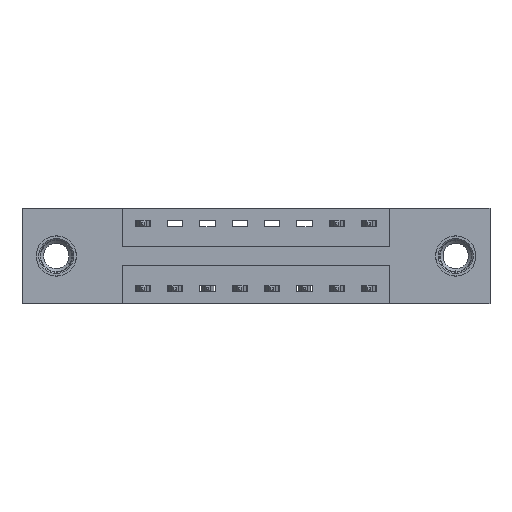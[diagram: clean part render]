
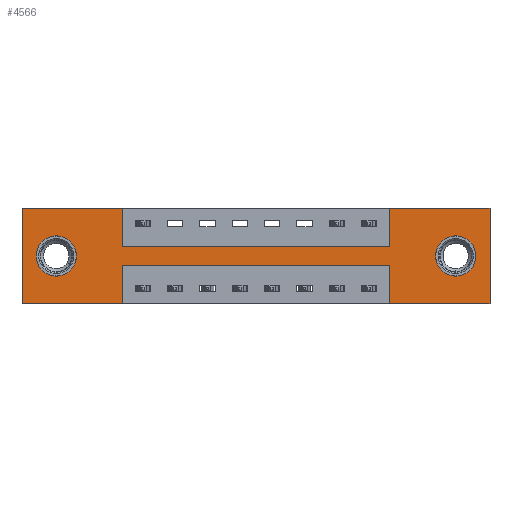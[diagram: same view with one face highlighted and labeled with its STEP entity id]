
A CAD part, front view. The second image highlights one B-rep face of the part: STEP entity #4566.
In plain terms, the highlighted planar face has unit normal (0, -1, 0).
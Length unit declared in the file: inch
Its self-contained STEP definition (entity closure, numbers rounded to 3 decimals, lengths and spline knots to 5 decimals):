
#24 = DIRECTION ( 'NONE',  ( 0., 0., -1. ) ) ;
#69 = DIRECTION ( 'NONE',  ( 0., 0., 1. ) ) ;
#92 = EDGE_CURVE ( 'NONE', #4048, #4417, #8899, .T. ) ;
#182 = CARTESIAN_POINT ( 'NONE',  ( 1.4225, 0., -0.15 ) ) ;
#255 = ORIENTED_EDGE ( 'NONE', *, *, #9028, .F. ) ;
#522 = VECTOR ( 'NONE', #6931, 39.37008 ) ;
#584 = VERTEX_POINT ( 'NONE', #8476 ) ;
#588 = DIRECTION ( 'NONE',  ( 0., 0., -1. ) ) ;
#597 = CARTESIAN_POINT ( 'NONE',  ( 1.6775, 0., -0.107 ) ) ;
#667 = ORIENTED_EDGE ( 'NONE', *, *, #2666, .F. ) ;
#691 = DIRECTION ( 'NONE',  ( 0., 0., 1. ) ) ;
#806 = DIRECTION ( 'NONE',  ( -1., 0., 0. ) ) ;
#878 = CARTESIAN_POINT ( 'NONE',  ( 0.1325, 0., -0.185 ) ) ;
#986 = FACE_OUTER_BOUND ( 'NONE', #8936, .T. ) ;
#999 = CARTESIAN_POINT ( 'NONE',  ( 1.4225, 0., -0.37 ) ) ;
#1041 = DIRECTION ( 'NONE',  ( -1., 0., 0. ) ) ;
#1147 = VERTEX_POINT ( 'NONE', #4420 ) ;
#1195 = DIRECTION ( 'NONE',  ( 1., 0., 0. ) ) ;
#1270 = CARTESIAN_POINT ( 'NONE',  ( 1.4225, 0., 0. ) ) ;
#1328 = LINE ( 'NONE', #5166, #9951 ) ;
#1451 = LINE ( 'NONE', #9693, #5874 ) ;
#1571 = FACE_BOUND ( 'NONE', #4125, .T. ) ;
#1792 = DIRECTION ( 'NONE',  ( 0., 0., 1. ) ) ;
#1912 = CARTESIAN_POINT ( 'NONE',  ( 1.81, 0., 0. ) ) ;
#1940 = VERTEX_POINT ( 'NONE', #2311 ) ;
#1969 = DIRECTION ( 'NONE',  ( 0., -1., 0. ) ) ;
#1970 = ORIENTED_EDGE ( 'NONE', *, *, #4651, .F. ) ;
#2231 = DIRECTION ( 'NONE',  ( 0., 0., -1. ) ) ;
#2251 = ORIENTED_EDGE ( 'NONE', *, *, #8188, .F. ) ;
#2311 = CARTESIAN_POINT ( 'NONE',  ( 0.1325, 0., -0.107 ) ) ;
#2666 = EDGE_CURVE ( 'NONE', #3934, #1147, #8643, .T. ) ;
#2674 = CARTESIAN_POINT ( 'NONE',  ( 0., 0., 0. ) ) ;
#2688 = CARTESIAN_POINT ( 'NONE',  ( 1.81, 0., 0. ) ) ;
#3094 = ORIENTED_EDGE ( 'NONE', *, *, #8072, .T. ) ;
#3206 = EDGE_CURVE ( 'NONE', #584, #7445, #9226, .T. ) ;
#3356 = AXIS2_PLACEMENT_3D ( 'NONE', #878, #6961, #1792 ) ;
#3616 = DIRECTION ( 'NONE',  ( 0., 0., -1. ) ) ;
#3652 = EDGE_CURVE ( 'NONE', #1147, #9329, #4982, .T. ) ;
#3721 = VERTEX_POINT ( 'NONE', #182 ) ;
#3740 = ORIENTED_EDGE ( 'NONE', *, *, #92, .F. ) ;
#3747 = AXIS2_PLACEMENT_3D ( 'NONE', #10166, #5443, #69 ) ;
#3749 = LINE ( 'NONE', #9170, #8137 ) ;
#3753 = CARTESIAN_POINT ( 'NONE',  ( 0.3875, 0., -0.22 ) ) ;
#3787 = CARTESIAN_POINT ( 'NONE',  ( 0., 0., -0.37 ) ) ;
#3835 = VERTEX_POINT ( 'NONE', #5760 ) ;
#3934 = VERTEX_POINT ( 'NONE', #8374 ) ;
#4048 = VERTEX_POINT ( 'NONE', #1912 ) ;
#4081 = VECTOR ( 'NONE', #3616, 39.37008 ) ;
#4125 = EDGE_LOOP ( 'NONE', ( #9941, #8256 ) ) ;
#4154 = CIRCLE ( 'NONE', #3747, 0.078 ) ;
#4271 = DIRECTION ( 'NONE',  ( 0., 1., 0. ) ) ;
#4306 = VECTOR ( 'NONE', #7866, 39.37008 ) ;
#4415 = CARTESIAN_POINT ( 'NONE',  ( 1.81, 0., -0.37 ) ) ;
#4417 = VERTEX_POINT ( 'NONE', #4415 ) ;
#4420 = CARTESIAN_POINT ( 'NONE',  ( 0.3875, 0., 0. ) ) ;
#4431 = VECTOR ( 'NONE', #24, 39.37008 ) ;
#4566 = ADVANCED_FACE ( 'NONE', ( #5719, #1571, #986 ), #9475, .T. ) ;
#4651 = EDGE_CURVE ( 'NONE', #3721, #7153, #6582, .T. ) ;
#4714 = DIRECTION ( 'NONE',  ( 1., 0., 0. ) ) ;
#4905 = ORIENTED_EDGE ( 'NONE', *, *, #5644, .F. ) ;
#4982 = LINE ( 'NONE', #9378, #4431 ) ;
#5100 = EDGE_LOOP ( 'NONE', ( #6902, #3094 ) ) ;
#5166 = CARTESIAN_POINT ( 'NONE',  ( 0., 0., -0.37 ) ) ;
#5443 = DIRECTION ( 'NONE',  ( 0., 1., 0. ) ) ;
#5510 = VECTOR ( 'NONE', #806, 39.37008 ) ;
#5639 = CARTESIAN_POINT ( 'NONE',  ( 0.3875, 0., -0.15 ) ) ;
#5644 = EDGE_CURVE ( 'NONE', #7153, #4048, #7439, .T. ) ;
#5719 = FACE_BOUND ( 'NONE', #5100, .T. ) ;
#5760 = CARTESIAN_POINT ( 'NONE',  ( 0.3875, 0., -0.37 ) ) ;
#5811 = ORIENTED_EDGE ( 'NONE', *, *, #10298, .F. ) ;
#5830 = ORIENTED_EDGE ( 'NONE', *, *, #3652, .F. ) ;
#5874 = VECTOR ( 'NONE', #2231, 39.37008 ) ;
#5878 = AXIS2_PLACEMENT_3D ( 'NONE', #3787, #1969, #7925 ) ;
#5919 = DIRECTION ( 'NONE',  ( 0., 1., 0. ) ) ;
#5929 = CARTESIAN_POINT ( 'NONE',  ( 1.4225, 0., 0. ) ) ;
#5945 = EDGE_CURVE ( 'NONE', #9329, #3721, #7047, .T. ) ;
#6000 = ORIENTED_EDGE ( 'NONE', *, *, #5945, .F. ) ;
#6213 = EDGE_CURVE ( 'NONE', #9638, #8257, #8794, .T. ) ;
#6582 = LINE ( 'NONE', #1270, #6834 ) ;
#6834 = VECTOR ( 'NONE', #7292, 39.37008 ) ;
#6902 = ORIENTED_EDGE ( 'NONE', *, *, #6213, .T. ) ;
#6931 = DIRECTION ( 'NONE',  ( 1., 0., 0. ) ) ;
#6961 = DIRECTION ( 'NONE',  ( 0., 1., 0. ) ) ;
#7005 = CIRCLE ( 'NONE', #7142, 0.078 ) ;
#7047 = LINE ( 'NONE', #5639, #8924 ) ;
#7110 = VECTOR ( 'NONE', #1041, 39.37008 ) ;
#7142 = AXIS2_PLACEMENT_3D ( 'NONE', #9103, #4271, #9871 ) ;
#7153 = VERTEX_POINT ( 'NONE', #5929 ) ;
#7172 = CARTESIAN_POINT ( 'NONE',  ( 0.3875, 0., -0.15 ) ) ;
#7292 = DIRECTION ( 'NONE',  ( 0., 0., 1. ) ) ;
#7439 = LINE ( 'NONE', #2674, #522 ) ;
#7445 = VERTEX_POINT ( 'NONE', #7760 ) ;
#7760 = CARTESIAN_POINT ( 'NONE',  ( 0.3875, 0., -0.22 ) ) ;
#7765 = CARTESIAN_POINT ( 'NONE',  ( 1.4225, 0., -0.37 ) ) ;
#7866 = DIRECTION ( 'NONE',  ( 0., 0., 1. ) ) ;
#7925 = DIRECTION ( 'NONE',  ( 0., 0., -1. ) ) ;
#8072 = EDGE_CURVE ( 'NONE', #8257, #9638, #7005, .T. ) ;
#8137 = VECTOR ( 'NONE', #691, 39.37008 ) ;
#8165 = EDGE_CURVE ( 'NONE', #3835, #9545, #1328, .T. ) ;
#8188 = EDGE_CURVE ( 'NONE', #9545, #3934, #3749, .T. ) ;
#8256 = ORIENTED_EDGE ( 'NONE', *, *, #10789, .T. ) ;
#8257 = VERTEX_POINT ( 'NONE', #9228 ) ;
#8342 = ORIENTED_EDGE ( 'NONE', *, *, #8165, .F. ) ;
#8374 = CARTESIAN_POINT ( 'NONE',  ( 0., 0., 0. ) ) ;
#8476 = CARTESIAN_POINT ( 'NONE',  ( 1.4225, 0., -0.22 ) ) ;
#8643 = LINE ( 'NONE', #10262, #8877 ) ;
#8794 = CIRCLE ( 'NONE', #10361, 0.078 ) ;
#8859 = LINE ( 'NONE', #999, #4306 ) ;
#8877 = VECTOR ( 'NONE', #4714, 39.37008 ) ;
#8899 = LINE ( 'NONE', #2688, #4081 ) ;
#8924 = VECTOR ( 'NONE', #1195, 39.37008 ) ;
#8936 = EDGE_LOOP ( 'NONE', ( #5811, #9159, #9221, #255, #3740, #4905, #1970, #6000, #5830, #667, #2251, #8342 ) ) ;
#8990 = VERTEX_POINT ( 'NONE', #10634 ) ;
#9028 = EDGE_CURVE ( 'NONE', #4417, #9861, #9708, .T. ) ;
#9103 = CARTESIAN_POINT ( 'NONE',  ( 1.6775, 0., -0.185 ) ) ;
#9159 = ORIENTED_EDGE ( 'NONE', *, *, #3206, .F. ) ;
#9170 = CARTESIAN_POINT ( 'NONE',  ( 0., 0., 0. ) ) ;
#9221 = ORIENTED_EDGE ( 'NONE', *, *, #9969, .F. ) ;
#9226 = LINE ( 'NONE', #3753, #7110 ) ;
#9228 = CARTESIAN_POINT ( 'NONE',  ( 1.6775, 0., -0.263 ) ) ;
#9329 = VERTEX_POINT ( 'NONE', #7172 ) ;
#9378 = CARTESIAN_POINT ( 'NONE',  ( 0.3875, 0., 0. ) ) ;
#9475 = PLANE ( 'NONE',  #5878 ) ;
#9545 = VERTEX_POINT ( 'NONE', #10496 ) ;
#9638 = VERTEX_POINT ( 'NONE', #597 ) ;
#9693 = CARTESIAN_POINT ( 'NONE',  ( 0.3875, 0., -0.37 ) ) ;
#9708 = LINE ( 'NONE', #10791, #5510 ) ;
#9826 = CIRCLE ( 'NONE', #3356, 0.078 ) ;
#9841 = EDGE_CURVE ( 'NONE', #1940, #8990, #9826, .T. ) ;
#9861 = VERTEX_POINT ( 'NONE', #7765 ) ;
#9871 = DIRECTION ( 'NONE',  ( 0., 0., -1. ) ) ;
#9941 = ORIENTED_EDGE ( 'NONE', *, *, #9841, .T. ) ;
#9951 = VECTOR ( 'NONE', #10701, 39.37008 ) ;
#9969 = EDGE_CURVE ( 'NONE', #9861, #584, #8859, .T. ) ;
#10166 = CARTESIAN_POINT ( 'NONE',  ( 0.1325, 0., -0.185 ) ) ;
#10262 = CARTESIAN_POINT ( 'NONE',  ( 0., 0., 0. ) ) ;
#10298 = EDGE_CURVE ( 'NONE', #7445, #3835, #1451, .T. ) ;
#10361 = AXIS2_PLACEMENT_3D ( 'NONE', #10621, #5919, #588 ) ;
#10496 = CARTESIAN_POINT ( 'NONE',  ( 0., 0., -0.37 ) ) ;
#10621 = CARTESIAN_POINT ( 'NONE',  ( 1.6775, 0., -0.185 ) ) ;
#10634 = CARTESIAN_POINT ( 'NONE',  ( 0.1325, 0., -0.263 ) ) ;
#10701 = DIRECTION ( 'NONE',  ( -1., 0., 0. ) ) ;
#10789 = EDGE_CURVE ( 'NONE', #8990, #1940, #4154, .T. ) ;
#10791 = CARTESIAN_POINT ( 'NONE',  ( 0., 0., -0.37 ) ) ;
